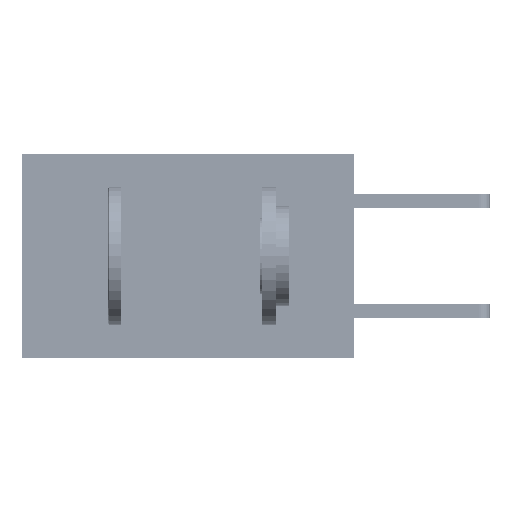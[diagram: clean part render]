
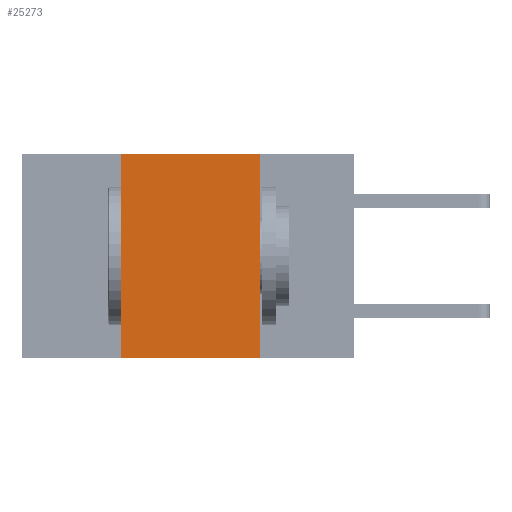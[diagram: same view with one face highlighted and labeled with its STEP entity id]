
A CAD part, left-side view. The second image highlights one B-rep face of the part: STEP entity #25273.
In plain terms, the highlighted planar face has unit normal (-1, 0, 0).
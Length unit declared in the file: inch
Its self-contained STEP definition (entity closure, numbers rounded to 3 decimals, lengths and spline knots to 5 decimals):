
#1180 = EDGE_CURVE ( 'NONE', #39964, #36163, #28010, .T. ) ;
#4598 = CARTESIAN_POINT ( 'NONE',  ( 0., 0.17, 0. ) ) ;
#4799 = PLANE ( 'NONE',  #7270 ) ;
#6958 = ORIENTED_EDGE ( 'NONE', *, *, #1180, .F. ) ;
#7270 = AXIS2_PLACEMENT_3D ( 'NONE', #31165, #8438, #41927 ) ;
#7949 = FACE_OUTER_BOUND ( 'NONE', #7989, .T. ) ;
#7989 = EDGE_LOOP ( 'NONE', ( #20989, #31071, #6958, #25245 ) ) ;
#8438 = DIRECTION ( 'NONE',  ( 1., 0., 0. ) ) ;
#8786 = CARTESIAN_POINT ( 'NONE',  ( 0., 0.42, 0. ) ) ;
#14522 = CARTESIAN_POINT ( 'NONE',  ( 0., 0.17, -0.37 ) ) ;
#16287 = VECTOR ( 'NONE', #24297, 39.37008 ) ;
#16337 = VECTOR ( 'NONE', #47431, 39.37008 ) ;
#17769 = EDGE_CURVE ( 'NONE', #22201, #23374, #27562, .T. ) ;
#18572 = VECTOR ( 'NONE', #39875, 39.37008 ) ;
#20989 = ORIENTED_EDGE ( 'NONE', *, *, #17769, .F. ) ;
#21210 = CARTESIAN_POINT ( 'NONE',  ( 0., 0.6, -0.37 ) ) ;
#22201 = VERTEX_POINT ( 'NONE', #39025 ) ;
#23374 = VERTEX_POINT ( 'NONE', #14522 ) ;
#24135 = CARTESIAN_POINT ( 'NONE',  ( 0., 0.42, 0. ) ) ;
#24297 = DIRECTION ( 'NONE',  ( 0., 0., -1. ) ) ;
#24641 = CARTESIAN_POINT ( 'NONE',  ( 0., 0.6, 0. ) ) ;
#25245 = ORIENTED_EDGE ( 'NONE', *, *, #39006, .T. ) ;
#25273 = ADVANCED_FACE ( 'NONE', ( #7949 ), #4799, .F. ) ;
#27562 = LINE ( 'NONE', #4598, #16287 ) ;
#28010 = LINE ( 'NONE', #8786, #40670 ) ;
#28631 = EDGE_CURVE ( 'NONE', #36163, #22201, #43620, .T. ) ;
#31071 = ORIENTED_EDGE ( 'NONE', *, *, #28631, .F. ) ;
#31165 = CARTESIAN_POINT ( 'NONE',  ( 0., 0.6, 0. ) ) ;
#36163 = VERTEX_POINT ( 'NONE', #24135 ) ;
#39006 = EDGE_CURVE ( 'NONE', #39964, #23374, #39940, .T. ) ;
#39025 = CARTESIAN_POINT ( 'NONE',  ( 0., 0.17, 0. ) ) ;
#39515 = CARTESIAN_POINT ( 'NONE',  ( 0., 0.42, -0.37 ) ) ;
#39875 = DIRECTION ( 'NONE',  ( 0., -1., 0. ) ) ;
#39940 = LINE ( 'NONE', #21210, #16337 ) ;
#39964 = VERTEX_POINT ( 'NONE', #39515 ) ;
#40670 = VECTOR ( 'NONE', #42991, 39.37008 ) ;
#41927 = DIRECTION ( 'NONE',  ( 0., 0., -1. ) ) ;
#42991 = DIRECTION ( 'NONE',  ( 0., 0., 1. ) ) ;
#43620 = LINE ( 'NONE', #24641, #18572 ) ;
#47431 = DIRECTION ( 'NONE',  ( 0., -1., 0. ) ) ;
